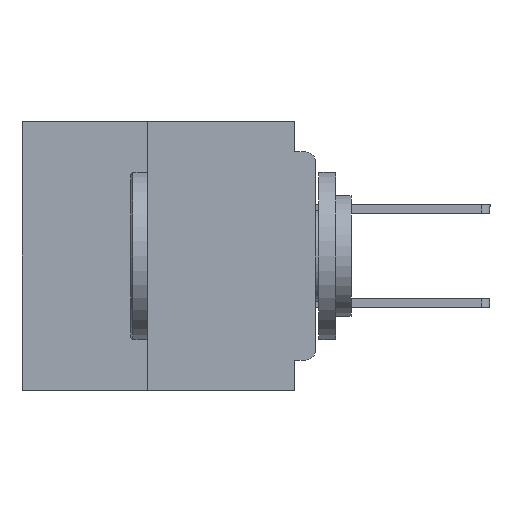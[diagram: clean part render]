
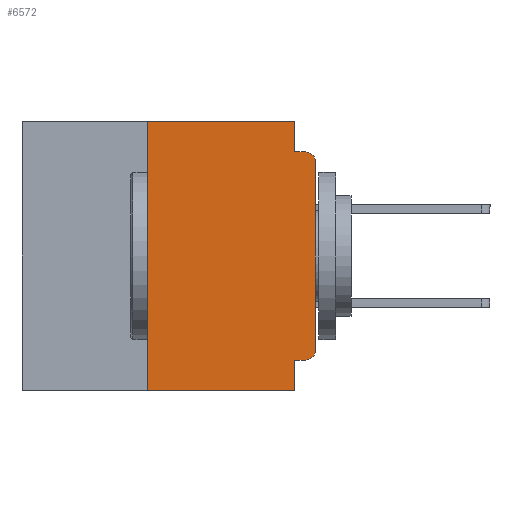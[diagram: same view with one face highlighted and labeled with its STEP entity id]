
A CAD part, left-side view. The second image highlights one B-rep face of the part: STEP entity #6572.
In plain terms, the highlighted planar face has unit normal (-1, 0, 0).
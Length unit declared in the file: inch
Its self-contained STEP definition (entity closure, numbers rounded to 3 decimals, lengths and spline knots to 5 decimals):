
#386 = EDGE_LOOP ( 'NONE', ( #14330, #44763, #29236, #42859, #25342, #28626, #32155, #1670, #40540, #26814 ) ) ;
#657 = VERTEX_POINT ( 'NONE', #48501 ) ;
#946 = DIRECTION ( 'NONE',  ( 0., 0., 1. ) ) ;
#1670 = ORIENTED_EDGE ( 'NONE', *, *, #34405, .F. ) ;
#2222 = VECTOR ( 'NONE', #11930, 39.37008 ) ;
#2244 = CARTESIAN_POINT ( 'NONE',  ( 0., 0.25, -0.4 ) ) ;
#2682 = VERTEX_POINT ( 'NONE', #37282 ) ;
#3565 = VERTEX_POINT ( 'NONE', #10163 ) ;
#4629 = VERTEX_POINT ( 'NONE', #9961 ) ;
#6572 = ADVANCED_FACE ( 'NONE', ( #11798 ), #14077, .F. ) ;
#6888 = LINE ( 'NONE', #20046, #48150 ) ;
#9537 = CARTESIAN_POINT ( 'NONE',  ( 0., 0.015, -0.045 ) ) ;
#9637 = DIRECTION ( 'NONE',  ( 0., 0., -1. ) ) ;
#9961 = CARTESIAN_POINT ( 'NONE',  ( 0., 0., -0.34 ) ) ;
#9997 = LINE ( 'NONE', #29327, #49907 ) ;
#10114 = CARTESIAN_POINT ( 'NONE',  ( 0., 0.031, -0.4 ) ) ;
#10138 = DIRECTION ( 'NONE',  ( 0., 1., 0. ) ) ;
#10163 = CARTESIAN_POINT ( 'NONE',  ( 0., 0.031, 0. ) ) ;
#10416 = DIRECTION ( 'NONE',  ( -1., 0., 0. ) ) ;
#10792 = CIRCLE ( 'NONE', #39693, 0.015 ) ;
#11798 = FACE_OUTER_BOUND ( 'NONE', #386, .T. ) ;
#11930 = DIRECTION ( 'NONE',  ( 0., -1., 0. ) ) ;
#11951 = LINE ( 'NONE', #21359, #42556 ) ;
#13140 = AXIS2_PLACEMENT_3D ( 'NONE', #34275, #10416, #38354 ) ;
#14077 = PLANE ( 'NONE',  #39762 ) ;
#14249 = DIRECTION ( 'NONE',  ( 0., 0., -1. ) ) ;
#14330 = ORIENTED_EDGE ( 'NONE', *, *, #51123, .T. ) ;
#14456 = CIRCLE ( 'NONE', #13140, 0.015 ) ;
#15217 = DIRECTION ( 'NONE',  ( 0., -1., 0. ) ) ;
#15669 = CARTESIAN_POINT ( 'NONE',  ( 0., 0.031, -0.045 ) ) ;
#17102 = VERTEX_POINT ( 'NONE', #10114 ) ;
#17615 = VERTEX_POINT ( 'NONE', #9537 ) ;
#18451 = EDGE_CURVE ( 'NONE', #25919, #17615, #10792, .T. ) ;
#20046 = CARTESIAN_POINT ( 'NONE',  ( 0., 0.437, -0.4 ) ) ;
#21359 = CARTESIAN_POINT ( 'NONE',  ( 0., 0.25, -0.4 ) ) ;
#21590 = CARTESIAN_POINT ( 'NONE',  ( 0., 0.031, -0.4 ) ) ;
#22299 = EDGE_CURVE ( 'NONE', #27507, #2682, #11951, .T. ) ;
#22788 = DIRECTION ( 'NONE',  ( -1., 0., 0. ) ) ;
#23068 = VERTEX_POINT ( 'NONE', #26281 ) ;
#23728 = LINE ( 'NONE', #35791, #2222 ) ;
#24013 = DIRECTION ( 'NONE',  ( 0., -1., 0. ) ) ;
#25342 = ORIENTED_EDGE ( 'NONE', *, *, #32036, .F. ) ;
#25553 = VECTOR ( 'NONE', #15217, 39.37008 ) ;
#25919 = VERTEX_POINT ( 'NONE', #33612 ) ;
#26060 = CARTESIAN_POINT ( 'NONE',  ( 0., 0.437, 0. ) ) ;
#26281 = CARTESIAN_POINT ( 'NONE',  ( 0., 0.031, -0.355 ) ) ;
#26814 = ORIENTED_EDGE ( 'NONE', *, *, #51880, .T. ) ;
#27446 = EDGE_CURVE ( 'NONE', #657, #23068, #40844, .T. ) ;
#27507 = VERTEX_POINT ( 'NONE', #2244 ) ;
#28626 = ORIENTED_EDGE ( 'NONE', *, *, #22299, .F. ) ;
#29236 = ORIENTED_EDGE ( 'NONE', *, *, #46696, .F. ) ;
#29327 = CARTESIAN_POINT ( 'NONE',  ( 0., 0., 0. ) ) ;
#30016 = CARTESIAN_POINT ( 'NONE',  ( 0., 0., -0.355 ) ) ;
#32036 = EDGE_CURVE ( 'NONE', #2682, #3565, #23728, .T. ) ;
#32155 = ORIENTED_EDGE ( 'NONE', *, *, #36352, .T. ) ;
#33302 = DIRECTION ( 'NONE',  ( 0., 0., 1. ) ) ;
#33612 = CARTESIAN_POINT ( 'NONE',  ( 0., 0., -0.06 ) ) ;
#34275 = CARTESIAN_POINT ( 'NONE',  ( 0., 0.015, -0.34 ) ) ;
#34405 = EDGE_CURVE ( 'NONE', #23068, #17102, #37142, .T. ) ;
#35791 = CARTESIAN_POINT ( 'NONE',  ( 0., 0.437, 0. ) ) ;
#36111 = LINE ( 'NONE', #50843, #25553 ) ;
#36292 = CARTESIAN_POINT ( 'NONE',  ( 0., 0.031, 0. ) ) ;
#36352 = EDGE_CURVE ( 'NONE', #27507, #17102, #6888, .T. ) ;
#37142 = LINE ( 'NONE', #21590, #47764 ) ;
#37282 = CARTESIAN_POINT ( 'NONE',  ( 0., 0.25, 0. ) ) ;
#37883 = VECTOR ( 'NONE', #40363, 39.37008 ) ;
#38084 = DIRECTION ( 'NONE',  ( 1., 0., 0. ) ) ;
#38354 = DIRECTION ( 'NONE',  ( 0., 0., -1. ) ) ;
#39693 = AXIS2_PLACEMENT_3D ( 'NONE', #46649, #22788, #50579 ) ;
#39762 = AXIS2_PLACEMENT_3D ( 'NONE', #26060, #38084, #14249 ) ;
#40363 = DIRECTION ( 'NONE',  ( 0., 0., -1. ) ) ;
#40540 = ORIENTED_EDGE ( 'NONE', *, *, #27446, .F. ) ;
#40844 = LINE ( 'NONE', #30016, #50110 ) ;
#41651 = VERTEX_POINT ( 'NONE', #15669 ) ;
#42556 = VECTOR ( 'NONE', #946, 39.37008 ) ;
#42859 = ORIENTED_EDGE ( 'NONE', *, *, #42912, .F. ) ;
#42912 = EDGE_CURVE ( 'NONE', #3565, #41651, #47243, .T. ) ;
#44763 = ORIENTED_EDGE ( 'NONE', *, *, #18451, .T. ) ;
#46649 = CARTESIAN_POINT ( 'NONE',  ( 0., 0.015, -0.06 ) ) ;
#46696 = EDGE_CURVE ( 'NONE', #41651, #17615, #36111, .T. ) ;
#47243 = LINE ( 'NONE', #36292, #37883 ) ;
#47764 = VECTOR ( 'NONE', #9637, 39.37008 ) ;
#48150 = VECTOR ( 'NONE', #24013, 39.37008 ) ;
#48501 = CARTESIAN_POINT ( 'NONE',  ( 0., 0.015, -0.355 ) ) ;
#49907 = VECTOR ( 'NONE', #33302, 39.37008 ) ;
#50110 = VECTOR ( 'NONE', #10138, 39.37008 ) ;
#50579 = DIRECTION ( 'NONE',  ( 0., 0., -1. ) ) ;
#50843 = CARTESIAN_POINT ( 'NONE',  ( 0., 0., -0.045 ) ) ;
#51123 = EDGE_CURVE ( 'NONE', #4629, #25919, #9997, .T. ) ;
#51880 = EDGE_CURVE ( 'NONE', #657, #4629, #14456, .T. ) ;
